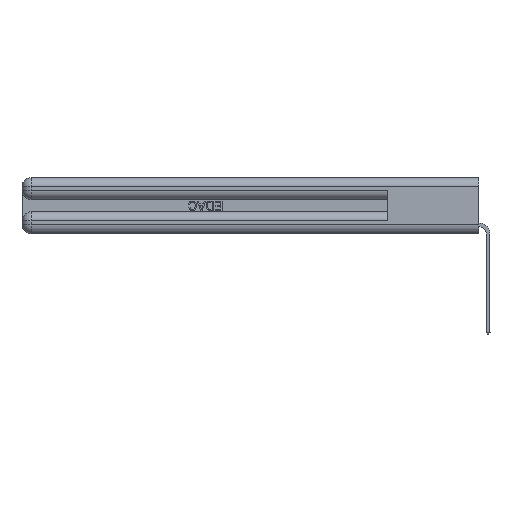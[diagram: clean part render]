
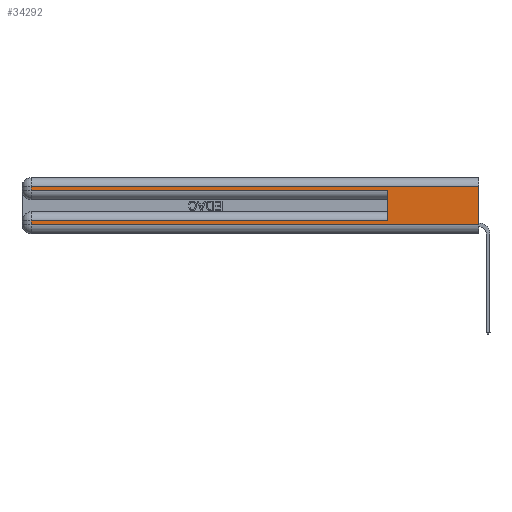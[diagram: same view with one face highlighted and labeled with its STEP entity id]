
A CAD part, left-side view. The second image highlights one B-rep face of the part: STEP entity #34292.
In plain terms, the highlighted planar face has unit normal (-1, 0, 0).
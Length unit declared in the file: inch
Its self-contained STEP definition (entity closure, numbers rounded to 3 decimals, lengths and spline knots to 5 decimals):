
#341 = CARTESIAN_POINT ( 'NONE',  ( 0., 0., 0.37 ) ) ;
#511 = VECTOR ( 'NONE', #29155, 39.37008 ) ;
#1374 = LINE ( 'NONE', #4671, #511 ) ;
#1598 = DIRECTION ( 'NONE',  ( 0., 1., 0. ) ) ;
#1820 = CARTESIAN_POINT ( 'NONE',  ( 0., 2.94, 0.06 ) ) ;
#2739 = LINE ( 'NONE', #31425, #9117 ) ;
#3412 = ORIENTED_EDGE ( 'NONE', *, *, #14203, .T. ) ;
#3976 = VECTOR ( 'NONE', #19327, 39.37008 ) ;
#4220 = VECTOR ( 'NONE', #6716, 39.37008 ) ;
#4671 = CARTESIAN_POINT ( 'NONE',  ( 0., 2.94, 0.37 ) ) ;
#6336 = CARTESIAN_POINT ( 'NONE',  ( 0., 0., 0.06 ) ) ;
#6716 = DIRECTION ( 'NONE',  ( 0., 0., -1. ) ) ;
#7326 = VECTOR ( 'NONE', #26747, 39.37008 ) ;
#7769 = CARTESIAN_POINT ( 'NONE',  ( 0., 0.6, 0.085 ) ) ;
#7867 = EDGE_CURVE ( 'NONE', #16291, #10838, #21233, .T. ) ;
#7964 = CARTESIAN_POINT ( 'NONE',  ( 0., 0.6, 0.285 ) ) ;
#8457 = VERTEX_POINT ( 'NONE', #12131 ) ;
#9027 = LINE ( 'NONE', #29499, #7326 ) ;
#9117 = VECTOR ( 'NONE', #1598, 39.37008 ) ;
#9234 = CARTESIAN_POINT ( 'NONE',  ( 0., 0., 0.37 ) ) ;
#9513 = ORIENTED_EDGE ( 'NONE', *, *, #34130, .F. ) ;
#10838 = VERTEX_POINT ( 'NONE', #25750 ) ;
#11153 = ORIENTED_EDGE ( 'NONE', *, *, #34994, .T. ) ;
#11979 = DIRECTION ( 'NONE',  ( 0., 0., -1. ) ) ;
#12131 = CARTESIAN_POINT ( 'NONE',  ( 0., 2.94, 0.285 ) ) ;
#12376 = VERTEX_POINT ( 'NONE', #19329 ) ;
#12475 = FACE_OUTER_BOUND ( 'NONE', #25960, .T. ) ;
#14019 = VECTOR ( 'NONE', #30826, 39.37008 ) ;
#14203 = EDGE_CURVE ( 'NONE', #12376, #8457, #26751, .T. ) ;
#14492 = CARTESIAN_POINT ( 'NONE',  ( 0., 0.6, 0.145 ) ) ;
#16291 = VERTEX_POINT ( 'NONE', #1820 ) ;
#16794 = EDGE_CURVE ( 'NONE', #21369, #33359, #33801, .T. ) ;
#17455 = ORIENTED_EDGE ( 'NONE', *, *, #7867, .T. ) ;
#17949 = ORIENTED_EDGE ( 'NONE', *, *, #35149, .T. ) ;
#18022 = CARTESIAN_POINT ( 'NONE',  ( 0., 0., 0.31 ) ) ;
#19327 = DIRECTION ( 'NONE',  ( 0., 0., -1. ) ) ;
#19329 = CARTESIAN_POINT ( 'NONE',  ( 0., 2.94, 0.31 ) ) ;
#19586 = AXIS2_PLACEMENT_3D ( 'NONE', #9234, #28271, #11979 ) ;
#20340 = CARTESIAN_POINT ( 'NONE',  ( 0., 0., 0.285 ) ) ;
#21233 = LINE ( 'NONE', #6336, #14019 ) ;
#21369 = VERTEX_POINT ( 'NONE', #7769 ) ;
#21878 = VERTEX_POINT ( 'NONE', #33884 ) ;
#22415 = ORIENTED_EDGE ( 'NONE', *, *, #16794, .F. ) ;
#22747 = PLANE ( 'NONE',  #19586 ) ;
#23072 = DIRECTION ( 'NONE',  ( 0., -1., 0. ) ) ;
#23909 = ORIENTED_EDGE ( 'NONE', *, *, #25075, .T. ) ;
#24491 = VERTEX_POINT ( 'NONE', #18022 ) ;
#24791 = LINE ( 'NONE', #341, #3976 ) ;
#25075 = EDGE_CURVE ( 'NONE', #24491, #12376, #2739, .T. ) ;
#25712 = CARTESIAN_POINT ( 'NONE',  ( 0., 2.94, 0.37 ) ) ;
#25750 = CARTESIAN_POINT ( 'NONE',  ( 0., 0., 0.06 ) ) ;
#25960 = EDGE_LOOP ( 'NONE', ( #9513, #23909, #3412, #11153, #22415, #32080, #17949, #17455 ) ) ;
#26747 = DIRECTION ( 'NONE',  ( 0., 1., 0. ) ) ;
#26751 = LINE ( 'NONE', #25712, #4220 ) ;
#27119 = EDGE_CURVE ( 'NONE', #21369, #21878, #9027, .T. ) ;
#27290 = VECTOR ( 'NONE', #23072, 39.37008 ) ;
#28175 = LINE ( 'NONE', #20340, #27290 ) ;
#28271 = DIRECTION ( 'NONE',  ( 1., 0., 0. ) ) ;
#29155 = DIRECTION ( 'NONE',  ( 0., 0., -1. ) ) ;
#29499 = CARTESIAN_POINT ( 'NONE',  ( 0., 0., 0.085 ) ) ;
#30791 = DIRECTION ( 'NONE',  ( 0., 0., 1. ) ) ;
#30826 = DIRECTION ( 'NONE',  ( 0., -1., 0. ) ) ;
#31425 = CARTESIAN_POINT ( 'NONE',  ( 0., 0., 0.31 ) ) ;
#32080 = ORIENTED_EDGE ( 'NONE', *, *, #27119, .T. ) ;
#32956 = VECTOR ( 'NONE', #30791, 39.37008 ) ;
#33359 = VERTEX_POINT ( 'NONE', #7964 ) ;
#33801 = LINE ( 'NONE', #14492, #32956 ) ;
#33884 = CARTESIAN_POINT ( 'NONE',  ( 0., 2.94, 0.085 ) ) ;
#34130 = EDGE_CURVE ( 'NONE', #24491, #10838, #24791, .T. ) ;
#34292 = ADVANCED_FACE ( 'NONE', ( #12475 ), #22747, .F. ) ;
#34994 = EDGE_CURVE ( 'NONE', #8457, #33359, #28175, .T. ) ;
#35149 = EDGE_CURVE ( 'NONE', #21878, #16291, #1374, .T. ) ;
